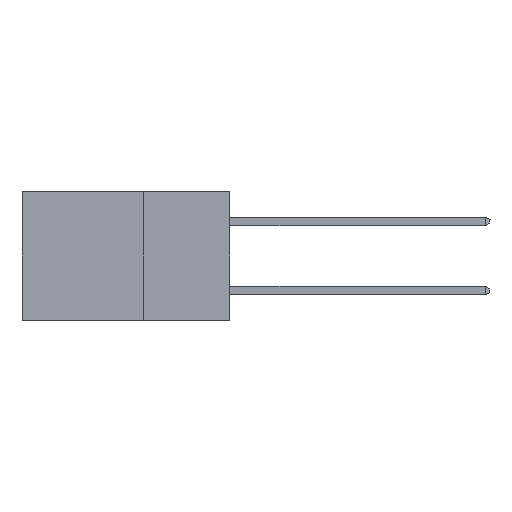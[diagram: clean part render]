
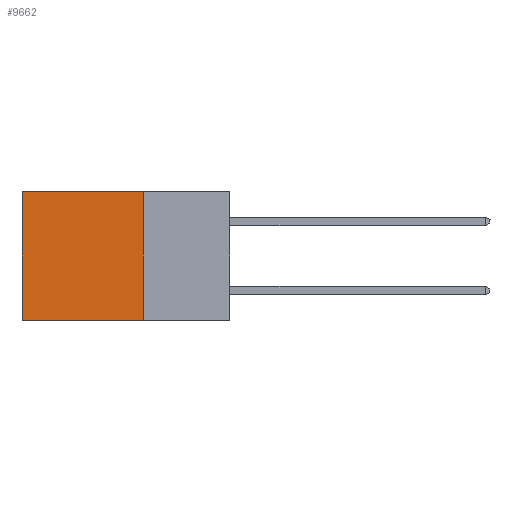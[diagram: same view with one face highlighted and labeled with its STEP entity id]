
A CAD part, left-side view. The second image highlights one B-rep face of the part: STEP entity #9662.
In plain terms, the highlighted planar face has unit normal (-1, 0, 0).
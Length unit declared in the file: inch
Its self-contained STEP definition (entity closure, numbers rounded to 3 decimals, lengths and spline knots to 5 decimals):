
#734 = FACE_OUTER_BOUND ( 'NONE', #25231, .T. ) ;
#2064 = VERTEX_POINT ( 'NONE', #8183 ) ;
#2332 = DIRECTION ( 'NONE',  ( 0., 1., 0. ) ) ;
#2912 = ORIENTED_EDGE ( 'NONE', *, *, #3235, .F. ) ;
#2913 = EDGE_CURVE ( 'NONE', #24466, #14159, #5063, .T. ) ;
#3087 = CARTESIAN_POINT ( 'NONE',  ( 0.298, 0.25, 0. ) ) ;
#3235 = EDGE_CURVE ( 'NONE', #14159, #2064, #23682, .T. ) ;
#4389 = VECTOR ( 'NONE', #15298, 39.37008 ) ;
#4472 = CARTESIAN_POINT ( 'NONE',  ( 0.298, 0.25, 0. ) ) ;
#5063 = LINE ( 'NONE', #12225, #4389 ) ;
#7403 = DIRECTION ( 'NONE',  ( 0., 0., -1. ) ) ;
#8183 = CARTESIAN_POINT ( 'NONE',  ( 0.298, 0.6, -0.37 ) ) ;
#8832 = ORIENTED_EDGE ( 'NONE', *, *, #2913, .F. ) ;
#9020 = VECTOR ( 'NONE', #26176, 39.37008 ) ;
#9662 = ADVANCED_FACE ( 'NONE', ( #734 ), #17468, .F. ) ;
#11109 = VERTEX_POINT ( 'NONE', #13585 ) ;
#12225 = CARTESIAN_POINT ( 'NONE',  ( 0.298, 0.25, 0. ) ) ;
#13585 = CARTESIAN_POINT ( 'NONE',  ( 0.298, 0.6, 0. ) ) ;
#14159 = VERTEX_POINT ( 'NONE', #23515 ) ;
#14168 = CARTESIAN_POINT ( 'NONE',  ( 0.298, 0.6, 0. ) ) ;
#14375 = LINE ( 'NONE', #14168, #9020 ) ;
#15298 = DIRECTION ( 'NONE',  ( 0., 0., -1. ) ) ;
#16408 = CARTESIAN_POINT ( 'NONE',  ( 0.298, 0.25, -0.37 ) ) ;
#16681 = DIRECTION ( 'NONE',  ( 0., 1., 0. ) ) ;
#16706 = VECTOR ( 'NONE', #2332, 39.37008 ) ;
#17468 = PLANE ( 'NONE',  #21882 ) ;
#17795 = VECTOR ( 'NONE', #16681, 39.37008 ) ;
#19444 = DIRECTION ( 'NONE',  ( 1., 0., 0. ) ) ;
#20872 = EDGE_CURVE ( 'NONE', #24466, #11109, #22203, .T. ) ;
#21882 = AXIS2_PLACEMENT_3D ( 'NONE', #3087, #19444, #7403 ) ;
#22203 = LINE ( 'NONE', #4472, #16706 ) ;
#22472 = EDGE_CURVE ( 'NONE', #11109, #2064, #14375, .T. ) ;
#23515 = CARTESIAN_POINT ( 'NONE',  ( 0.298, 0.25, -0.37 ) ) ;
#23682 = LINE ( 'NONE', #16408, #17795 ) ;
#23754 = ORIENTED_EDGE ( 'NONE', *, *, #20872, .T. ) ;
#23916 = CARTESIAN_POINT ( 'NONE',  ( 0.298, 0.25, 0. ) ) ;
#24466 = VERTEX_POINT ( 'NONE', #23916 ) ;
#24977 = ORIENTED_EDGE ( 'NONE', *, *, #22472, .T. ) ;
#25231 = EDGE_LOOP ( 'NONE', ( #24977, #2912, #8832, #23754 ) ) ;
#26176 = DIRECTION ( 'NONE',  ( 0., 0., -1. ) ) ;
